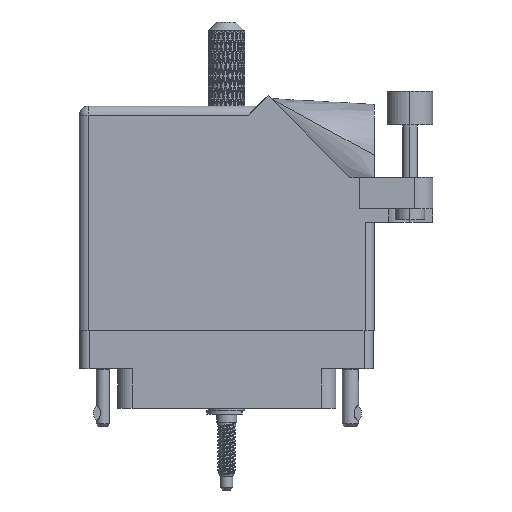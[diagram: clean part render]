
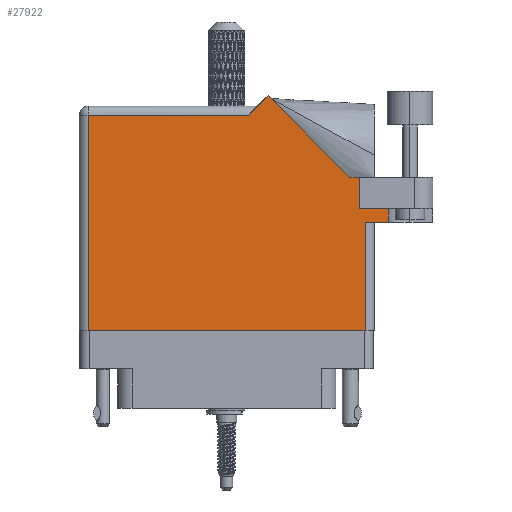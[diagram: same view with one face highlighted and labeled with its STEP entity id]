
A CAD part, front view. The second image highlights one B-rep face of the part: STEP entity #27922.
In plain terms, the highlighted face is planar.
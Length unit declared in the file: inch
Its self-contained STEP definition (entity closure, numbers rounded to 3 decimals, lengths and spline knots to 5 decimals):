
#501 = VECTOR ( 'NONE', #55171, 39.37008 ) ;
#2186 = DIRECTION ( 'NONE',  ( 0., -1., 0. ) ) ;
#2277 = DIRECTION ( 'NONE',  ( -1., 0., 0. ) ) ;
#2633 = CARTESIAN_POINT ( 'NONE',  ( 0.062, 0., 0. ) ) ;
#3240 = ORIENTED_EDGE ( 'NONE', *, *, #24726, .T. ) ;
#3371 = DIRECTION ( 'NONE',  ( -0.707, -0.707, 0. ) ) ;
#5635 = EDGE_CURVE ( 'NONE', #70071, #10947, #31619, .T. ) ;
#7007 = EDGE_CURVE ( 'NONE', #105273, #111780, #38256, .T. ) ;
#8386 = LINE ( 'NONE', #96406, #105546 ) ;
#9759 = LINE ( 'NONE', #110655, #60805 ) ;
#10808 = VERTEX_POINT ( 'NONE', #73534 ) ;
#10947 = VERTEX_POINT ( 'NONE', #95907 ) ;
#15468 = EDGE_CURVE ( 'NONE', #10808, #80142, #59373, .T. ) ;
#16794 = LINE ( 'NONE', #37472, #19505 ) ;
#17310 = EDGE_CURVE ( 'NONE', #80806, #105273, #98969, .T. ) ;
#17971 = CARTESIAN_POINT ( 'NONE',  ( 2.1115, 0.737, 0. ) ) ;
#17995 = DIRECTION ( 'NONE',  ( 1., 0., 0. ) ) ;
#18566 = DIRECTION ( 'NONE',  ( 0., 1., 0. ) ) ;
#19505 = VECTOR ( 'NONE', #107332, 39.37008 ) ;
#19616 = CARTESIAN_POINT ( 'NONE',  ( 0.062, 0., 0. ) ) ;
#24726 = EDGE_CURVE ( 'NONE', #104985, #103273, #103543, .T. ) ;
#26833 = AXIS2_PLACEMENT_3D ( 'NONE', #114235, #61365, #2277 ) ;
#27922 = ADVANCED_FACE ( 'NONE', ( #70957 ), #96472, .F. ) ;
#27928 = EDGE_CURVE ( 'NONE', #10947, #84273, #54345, .T. ) ;
#28616 = VECTOR ( 'NONE', #2186, 39.37008 ) ;
#30301 = EDGE_CURVE ( 'NONE', #80806, #10808, #58348, .T. ) ;
#31619 = LINE ( 'NONE', #76774, #62093 ) ;
#34275 = DIRECTION ( 'NONE',  ( 1., 0., 0. ) ) ;
#35796 = CARTESIAN_POINT ( 'NONE',  ( 1.28771, 1.60071, 0. ) ) ;
#36386 = CARTESIAN_POINT ( 'NONE',  ( 1.948, 0.737, 0. ) ) ;
#36696 = CARTESIAN_POINT ( 'NONE',  ( 1.948, 0., 0. ) ) ;
#37472 = CARTESIAN_POINT ( 'NONE',  ( 2.01, 0.737, 0. ) ) ;
#38256 = LINE ( 'NONE', #99383, #28616 ) ;
#44800 = CARTESIAN_POINT ( 'NONE',  ( 1.84442, 1.044, 0. ) ) ;
#47530 = CARTESIAN_POINT ( 'NONE',  ( 2.41, 1.044, 0. ) ) ;
#52363 = ORIENTED_EDGE ( 'NONE', *, *, #30301, .T. ) ;
#54345 = LINE ( 'NONE', #19616, #501 ) ;
#55171 = DIRECTION ( 'NONE',  ( 0., -1., 0. ) ) ;
#55437 = ORIENTED_EDGE ( 'NONE', *, *, #15468, .T. ) ;
#56196 = EDGE_CURVE ( 'NONE', #103273, #111780, #16794, .T. ) ;
#56292 = LINE ( 'NONE', #44800, #86608 ) ;
#56784 = VERTEX_POINT ( 'NONE', #35796 ) ;
#58348 = LINE ( 'NONE', #62216, #106475 ) ;
#59373 = LINE ( 'NONE', #47530, #85594 ) ;
#60805 = VECTOR ( 'NONE', #3371, 39.37008 ) ;
#61365 = DIRECTION ( 'NONE',  ( 0., 0., -1. ) ) ;
#62093 = VECTOR ( 'NONE', #67908, 39.37008 ) ;
#62216 = CARTESIAN_POINT ( 'NONE',  ( 1.91, 0.831, 0. ) ) ;
#62655 = ORIENTED_EDGE ( 'NONE', *, *, #27928, .T. ) ;
#64437 = EDGE_CURVE ( 'NONE', #80142, #56784, #56292, .T. ) ;
#65232 = EDGE_LOOP ( 'NONE', ( #69528, #3240, #79360, #84514, #74414, #52363, #55437, #74447, #111119, #97635, #62655 ) ) ;
#67908 = DIRECTION ( 'NONE',  ( -1., 0., 0. ) ) ;
#68010 = DIRECTION ( 'NONE',  ( -1., 0., 0. ) ) ;
#69528 = ORIENTED_EDGE ( 'NONE', *, *, #99755, .T. ) ;
#70071 = VERTEX_POINT ( 'NONE', #97055 ) ;
#70957 = FACE_OUTER_BOUND ( 'NONE', #65232, .T. ) ;
#71420 = DIRECTION ( 'NONE',  ( -0.707, 0.707, 0. ) ) ;
#73534 = CARTESIAN_POINT ( 'NONE',  ( 1.91, 1.044, 0. ) ) ;
#74414 = ORIENTED_EDGE ( 'NONE', *, *, #17310, .F. ) ;
#74447 = ORIENTED_EDGE ( 'NONE', *, *, #64437, .T. ) ;
#75521 = VECTOR ( 'NONE', #17995, 39.37008 ) ;
#76774 = CARTESIAN_POINT ( 'NONE',  ( 0., 1.468, 0. ) ) ;
#79360 = ORIENTED_EDGE ( 'NONE', *, *, #56196, .T. ) ;
#80142 = VERTEX_POINT ( 'NONE', #106608 ) ;
#80806 = VERTEX_POINT ( 'NONE', #103675 ) ;
#82263 = CARTESIAN_POINT ( 'NONE',  ( 1.948, 0.737, 0. ) ) ;
#84273 = VERTEX_POINT ( 'NONE', #2633 ) ;
#84514 = ORIENTED_EDGE ( 'NONE', *, *, #7007, .F. ) ;
#85594 = VECTOR ( 'NONE', #68010, 39.37008 ) ;
#86608 = VECTOR ( 'NONE', #71420, 39.37008 ) ;
#92510 = CARTESIAN_POINT ( 'NONE',  ( 1.91, 0.831, 0. ) ) ;
#95907 = CARTESIAN_POINT ( 'NONE',  ( 0.062, 1.468, 0. ) ) ;
#96406 = CARTESIAN_POINT ( 'NONE',  ( 0., 0., 0. ) ) ;
#96472 = PLANE ( 'NONE',  #26833 ) ;
#97055 = CARTESIAN_POINT ( 'NONE',  ( 1.155, 1.468, 0. ) ) ;
#97635 = ORIENTED_EDGE ( 'NONE', *, *, #5635, .T. ) ;
#98969 = LINE ( 'NONE', #92510, #75521 ) ;
#99383 = CARTESIAN_POINT ( 'NONE',  ( 2.1115, 1.16177, 0. ) ) ;
#99755 = EDGE_CURVE ( 'NONE', #84273, #104985, #8386, .T. ) ;
#103273 = VERTEX_POINT ( 'NONE', #82263 ) ;
#103543 = LINE ( 'NONE', #36386, #110448 ) ;
#103675 = CARTESIAN_POINT ( 'NONE',  ( 1.91, 0.831, 0. ) ) ;
#104342 = CARTESIAN_POINT ( 'NONE',  ( 2.1115, 0.831, 0. ) ) ;
#104985 = VERTEX_POINT ( 'NONE', #36696 ) ;
#105273 = VERTEX_POINT ( 'NONE', #104342 ) ;
#105546 = VECTOR ( 'NONE', #34275, 39.37008 ) ;
#106475 = VECTOR ( 'NONE', #18566, 39.37008 ) ;
#106608 = CARTESIAN_POINT ( 'NONE',  ( 1.84442, 1.044, 0. ) ) ;
#107009 = DIRECTION ( 'NONE',  ( 0., 1., 0. ) ) ;
#107332 = DIRECTION ( 'NONE',  ( 1., 0., 0. ) ) ;
#110448 = VECTOR ( 'NONE', #107009, 39.37008 ) ;
#110587 = EDGE_CURVE ( 'NONE', #56784, #70071, #9759, .T. ) ;
#110655 = CARTESIAN_POINT ( 'NONE',  ( 1.217, 1.53, 0. ) ) ;
#111119 = ORIENTED_EDGE ( 'NONE', *, *, #110587, .T. ) ;
#111780 = VERTEX_POINT ( 'NONE', #17971 ) ;
#114235 = CARTESIAN_POINT ( 'NONE',  ( 0., 1.53, 0. ) ) ;
